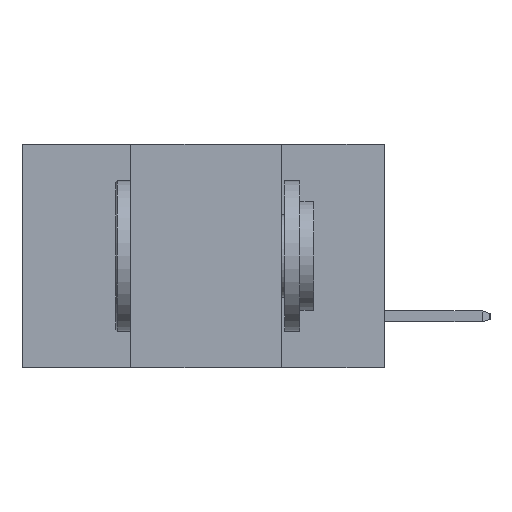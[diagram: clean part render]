
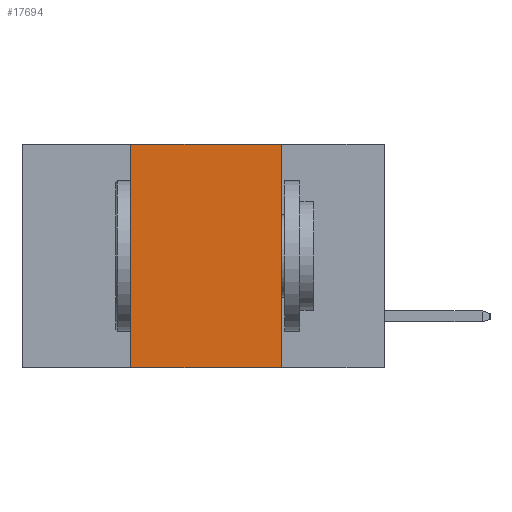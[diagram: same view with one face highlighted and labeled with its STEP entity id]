
A CAD part, left-side view. The second image highlights one B-rep face of the part: STEP entity #17694.
In plain terms, the highlighted planar face has unit normal (-1, 0, 0).
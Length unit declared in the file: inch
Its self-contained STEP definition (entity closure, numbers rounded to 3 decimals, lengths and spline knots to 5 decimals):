
#26 = CARTESIAN_POINT ( 'NONE',  ( 0., 0.42, -0.37 ) ) ;
#177 = AXIS2_PLACEMENT_3D ( 'NONE', #876, #12251, #2527 ) ;
#876 = CARTESIAN_POINT ( 'NONE',  ( 0., 0.6, 0. ) ) ;
#1111 = VECTOR ( 'NONE', #9642, 39.37008 ) ;
#1617 = LINE ( 'NONE', #8000, #1111 ) ;
#1827 = LINE ( 'NONE', #11930, #5185 ) ;
#1831 = VERTEX_POINT ( 'NONE', #26 ) ;
#2527 = DIRECTION ( 'NONE',  ( 0., 0., -1. ) ) ;
#3930 = ORIENTED_EDGE ( 'NONE', *, *, #10393, .T. ) ;
#3934 = CARTESIAN_POINT ( 'NONE',  ( 0., 0.42, 0. ) ) ;
#4011 = VERTEX_POINT ( 'NONE', #3934 ) ;
#5185 = VECTOR ( 'NONE', #13458, 39.37008 ) ;
#5582 = FACE_OUTER_BOUND ( 'NONE', #15539, .T. ) ;
#6873 = VERTEX_POINT ( 'NONE', #9452 ) ;
#8000 = CARTESIAN_POINT ( 'NONE',  ( 0., 0.17, -0.37 ) ) ;
#8320 = ORIENTED_EDGE ( 'NONE', *, *, #15456, .F. ) ;
#8435 = CARTESIAN_POINT ( 'NONE',  ( 0., 0.42, -0.37 ) ) ;
#9131 = PLANE ( 'NONE',  #177 ) ;
#9452 = CARTESIAN_POINT ( 'NONE',  ( 0., 0.17, 0. ) ) ;
#9642 = DIRECTION ( 'NONE',  ( 0., 0., -1. ) ) ;
#10066 = DIRECTION ( 'NONE',  ( 0., 0., 1. ) ) ;
#10393 = EDGE_CURVE ( 'NONE', #1831, #11610, #15557, .T. ) ;
#11223 = CARTESIAN_POINT ( 'NONE',  ( 0., 0.17, -0.37 ) ) ;
#11281 = LINE ( 'NONE', #8435, #18767 ) ;
#11563 = VECTOR ( 'NONE', #18778, 39.37008 ) ;
#11610 = VERTEX_POINT ( 'NONE', #11223 ) ;
#11930 = CARTESIAN_POINT ( 'NONE',  ( 0., 0.6, 0. ) ) ;
#12251 = DIRECTION ( 'NONE',  ( 1., 0., 0. ) ) ;
#13341 = EDGE_CURVE ( 'NONE', #6873, #11610, #1617, .T. ) ;
#13458 = DIRECTION ( 'NONE',  ( 0., -1., 0. ) ) ;
#14344 = EDGE_CURVE ( 'NONE', #4011, #6873, #1827, .T. ) ;
#15456 = EDGE_CURVE ( 'NONE', #1831, #4011, #11281, .T. ) ;
#15539 = EDGE_LOOP ( 'NONE', ( #16968, #16515, #8320, #3930 ) ) ;
#15557 = LINE ( 'NONE', #15799, #11563 ) ;
#15799 = CARTESIAN_POINT ( 'NONE',  ( 0., 0.6, -0.37 ) ) ;
#16515 = ORIENTED_EDGE ( 'NONE', *, *, #14344, .F. ) ;
#16968 = ORIENTED_EDGE ( 'NONE', *, *, #13341, .F. ) ;
#17694 = ADVANCED_FACE ( 'NONE', ( #5582 ), #9131, .F. ) ;
#18767 = VECTOR ( 'NONE', #10066, 39.37008 ) ;
#18778 = DIRECTION ( 'NONE',  ( 0., -1., 0. ) ) ;
